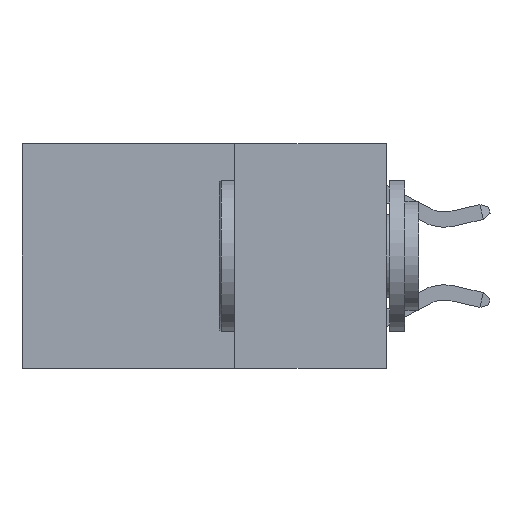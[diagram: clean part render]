
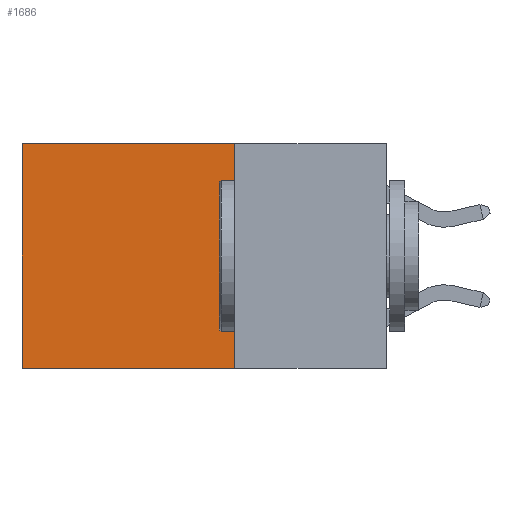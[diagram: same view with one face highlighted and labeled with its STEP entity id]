
A CAD part, left-side view. The second image highlights one B-rep face of the part: STEP entity #1686.
In plain terms, the highlighted planar face has unit normal (-1, 0, 0).
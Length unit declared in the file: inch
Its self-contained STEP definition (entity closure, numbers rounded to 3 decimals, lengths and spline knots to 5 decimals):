
#1686 = ADVANCED_FACE ( 'NONE', ( #28911 ), #23505, .F. ) ;
#3171 = ORIENTED_EDGE ( 'NONE', *, *, #4502, .T. ) ;
#4454 = DIRECTION ( 'NONE',  ( 0., 1., 0. ) ) ;
#4502 = EDGE_CURVE ( 'NONE', #12084, #11861, #29858, .T. ) ;
#5322 = LINE ( 'NONE', #28706, #30804 ) ;
#7263 = DIRECTION ( 'NONE',  ( 1., 0., 0. ) ) ;
#8954 = CARTESIAN_POINT ( 'NONE',  ( 0.2625, 0.6, -0.37 ) ) ;
#9102 = LINE ( 'NONE', #10904, #17196 ) ;
#9719 = CARTESIAN_POINT ( 'NONE',  ( 0.2625, 0.25, 0. ) ) ;
#9818 = LINE ( 'NONE', #10121, #15955 ) ;
#10121 = CARTESIAN_POINT ( 'NONE',  ( 0.2625, 0.25, -0.37 ) ) ;
#10904 = CARTESIAN_POINT ( 'NONE',  ( 0.2625, 0.25, 0. ) ) ;
#11174 = VERTEX_POINT ( 'NONE', #26650 ) ;
#11861 = VERTEX_POINT ( 'NONE', #24544 ) ;
#12084 = VERTEX_POINT ( 'NONE', #22933 ) ;
#12089 = DIRECTION ( 'NONE',  ( 0., 0., -1. ) ) ;
#13647 = VECTOR ( 'NONE', #4454, 39.37008 ) ;
#15955 = VECTOR ( 'NONE', #24957, 39.37008 ) ;
#16635 = CARTESIAN_POINT ( 'NONE',  ( 0.2625, 0.25, 0. ) ) ;
#16719 = EDGE_CURVE ( 'NONE', #12084, #11174, #9102, .T. ) ;
#16819 = ORIENTED_EDGE ( 'NONE', *, *, #16719, .F. ) ;
#16957 = ORIENTED_EDGE ( 'NONE', *, *, #21084, .T. ) ;
#17196 = VECTOR ( 'NONE', #20689, 39.37008 ) ;
#18726 = AXIS2_PLACEMENT_3D ( 'NONE', #9719, #7263, #12089 ) ;
#19693 = EDGE_LOOP ( 'NONE', ( #16957, #30888, #16819, #3171 ) ) ;
#20209 = VERTEX_POINT ( 'NONE', #8954 ) ;
#20689 = DIRECTION ( 'NONE',  ( 0., 0., -1. ) ) ;
#21084 = EDGE_CURVE ( 'NONE', #11861, #20209, #5322, .T. ) ;
#22933 = CARTESIAN_POINT ( 'NONE',  ( 0.2625, 0.25, 0. ) ) ;
#23505 = PLANE ( 'NONE',  #18726 ) ;
#24544 = CARTESIAN_POINT ( 'NONE',  ( 0.2625, 0.6, 0. ) ) ;
#24957 = DIRECTION ( 'NONE',  ( 0., 1., 0. ) ) ;
#26650 = CARTESIAN_POINT ( 'NONE',  ( 0.2625, 0.25, -0.37 ) ) ;
#28706 = CARTESIAN_POINT ( 'NONE',  ( 0.2625, 0.6, 0. ) ) ;
#28911 = FACE_OUTER_BOUND ( 'NONE', #19693, .T. ) ;
#29669 = EDGE_CURVE ( 'NONE', #11174, #20209, #9818, .T. ) ;
#29858 = LINE ( 'NONE', #16635, #13647 ) ;
#30804 = VECTOR ( 'NONE', #30857, 39.37008 ) ;
#30857 = DIRECTION ( 'NONE',  ( 0., 0., -1. ) ) ;
#30888 = ORIENTED_EDGE ( 'NONE', *, *, #29669, .F. ) ;
